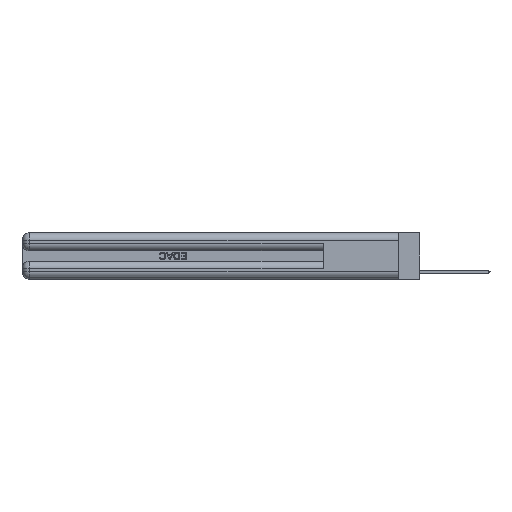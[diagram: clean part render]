
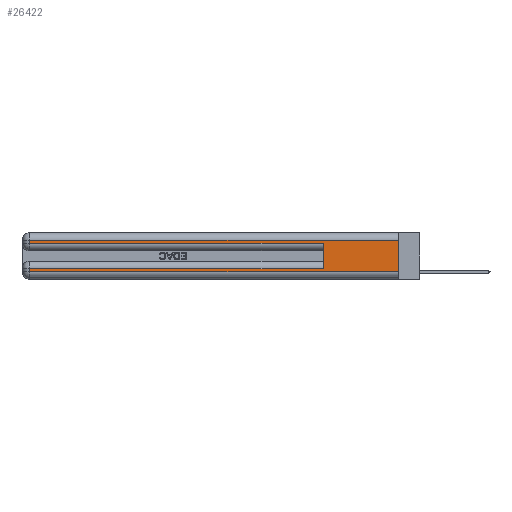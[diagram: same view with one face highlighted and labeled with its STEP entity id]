
A CAD part, left-side view. The second image highlights one B-rep face of the part: STEP entity #26422.
In plain terms, the highlighted planar face has unit normal (-1, 0, 0).
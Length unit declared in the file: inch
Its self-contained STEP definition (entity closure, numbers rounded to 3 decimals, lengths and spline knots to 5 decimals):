
#332 = ORIENTED_EDGE ( 'NONE', *, *, #34627, .T. ) ;
#1749 = CARTESIAN_POINT ( 'NONE',  ( 0., 2.94, 0.31 ) ) ;
#1881 = ORIENTED_EDGE ( 'NONE', *, *, #20156, .T. ) ;
#1884 = VERTEX_POINT ( 'NONE', #12785 ) ;
#2151 = ORIENTED_EDGE ( 'NONE', *, *, #9709, .T. ) ;
#2262 = CARTESIAN_POINT ( 'NONE',  ( 0., 2.94, 0.37 ) ) ;
#3121 = LINE ( 'NONE', #33482, #12870 ) ;
#4342 = VECTOR ( 'NONE', #13943, 39.37008 ) ;
#4448 = DIRECTION ( 'NONE',  ( 0., 0., -1. ) ) ;
#4853 = DIRECTION ( 'NONE',  ( 0., -1., 0. ) ) ;
#5162 = ORIENTED_EDGE ( 'NONE', *, *, #14232, .F. ) ;
#5972 = VERTEX_POINT ( 'NONE', #6393 ) ;
#6241 = VERTEX_POINT ( 'NONE', #8522 ) ;
#6393 = CARTESIAN_POINT ( 'NONE',  ( 0., 0.6, 0.085 ) ) ;
#7024 = VERTEX_POINT ( 'NONE', #1749 ) ;
#7501 = LINE ( 'NONE', #24125, #8134 ) ;
#7768 = CARTESIAN_POINT ( 'NONE',  ( 0., 0., 0.31 ) ) ;
#7909 = EDGE_LOOP ( 'NONE', ( #17252, #32436, #8553, #2151, #5162, #1881, #332, #27523 ) ) ;
#7910 = VECTOR ( 'NONE', #22847, 39.37008 ) ;
#8134 = VECTOR ( 'NONE', #8219, 39.37008 ) ;
#8219 = DIRECTION ( 'NONE',  ( 0., -1., 0. ) ) ;
#8522 = CARTESIAN_POINT ( 'NONE',  ( 0., 2.94, 0.285 ) ) ;
#8553 = ORIENTED_EDGE ( 'NONE', *, *, #19678, .T. ) ;
#9529 = CARTESIAN_POINT ( 'NONE',  ( 0., 0., 0.37 ) ) ;
#9709 = EDGE_CURVE ( 'NONE', #6241, #11532, #16618, .T. ) ;
#10298 = DIRECTION ( 'NONE',  ( 0., 1., 0. ) ) ;
#11532 = VERTEX_POINT ( 'NONE', #32826 ) ;
#12074 = FACE_OUTER_BOUND ( 'NONE', #7909, .T. ) ;
#12177 = LINE ( 'NONE', #31848, #17243 ) ;
#12514 = LINE ( 'NONE', #18135, #7910 ) ;
#12785 = CARTESIAN_POINT ( 'NONE',  ( 0., 0., 0.06 ) ) ;
#12870 = VECTOR ( 'NONE', #19405, 39.37008 ) ;
#13943 = DIRECTION ( 'NONE',  ( 0., 1., 0. ) ) ;
#14232 = EDGE_CURVE ( 'NONE', #5972, #11532, #3121, .T. ) ;
#14872 = VERTEX_POINT ( 'NONE', #17557 ) ;
#15787 = DIRECTION ( 'NONE',  ( 0., 0., -1. ) ) ;
#16210 = LINE ( 'NONE', #2262, #18440 ) ;
#16618 = LINE ( 'NONE', #32509, #30631 ) ;
#16631 = VERTEX_POINT ( 'NONE', #17161 ) ;
#17161 = CARTESIAN_POINT ( 'NONE',  ( 0., 2.94, 0.085 ) ) ;
#17243 = VECTOR ( 'NONE', #15787, 39.37008 ) ;
#17252 = ORIENTED_EDGE ( 'NONE', *, *, #24748, .F. ) ;
#17557 = CARTESIAN_POINT ( 'NONE',  ( 0., 2.94, 0.06 ) ) ;
#17682 = PLANE ( 'NONE',  #24805 ) ;
#18135 = CARTESIAN_POINT ( 'NONE',  ( 0., 2.94, 0.37 ) ) ;
#18204 = VERTEX_POINT ( 'NONE', #33874 ) ;
#18440 = VECTOR ( 'NONE', #21803, 39.37008 ) ;
#19405 = DIRECTION ( 'NONE',  ( 0., 0., 1. ) ) ;
#19549 = CARTESIAN_POINT ( 'NONE',  ( 0., 0., 0.085 ) ) ;
#19678 = EDGE_CURVE ( 'NONE', #7024, #6241, #16210, .T. ) ;
#20156 = EDGE_CURVE ( 'NONE', #5972, #16631, #33439, .T. ) ;
#21803 = DIRECTION ( 'NONE',  ( 0., 0., -1. ) ) ;
#22847 = DIRECTION ( 'NONE',  ( 0., 0., -1. ) ) ;
#23104 = DIRECTION ( 'NONE',  ( 1., 0., 0. ) ) ;
#24125 = CARTESIAN_POINT ( 'NONE',  ( 0., 0., 0.06 ) ) ;
#24748 = EDGE_CURVE ( 'NONE', #18204, #1884, #12177, .T. ) ;
#24805 = AXIS2_PLACEMENT_3D ( 'NONE', #9529, #23104, #4448 ) ;
#26422 = ADVANCED_FACE ( 'NONE', ( #12074 ), #17682, .F. ) ;
#27523 = ORIENTED_EDGE ( 'NONE', *, *, #28096, .T. ) ;
#28096 = EDGE_CURVE ( 'NONE', #14872, #1884, #7501, .T. ) ;
#29637 = LINE ( 'NONE', #7768, #31010 ) ;
#30631 = VECTOR ( 'NONE', #4853, 39.37008 ) ;
#31010 = VECTOR ( 'NONE', #10298, 39.37008 ) ;
#31848 = CARTESIAN_POINT ( 'NONE',  ( 0., 0., 0.37 ) ) ;
#32436 = ORIENTED_EDGE ( 'NONE', *, *, #35143, .T. ) ;
#32509 = CARTESIAN_POINT ( 'NONE',  ( 0., 0., 0.285 ) ) ;
#32826 = CARTESIAN_POINT ( 'NONE',  ( 0., 0.6, 0.285 ) ) ;
#33439 = LINE ( 'NONE', #19549, #4342 ) ;
#33482 = CARTESIAN_POINT ( 'NONE',  ( 0., 0.6, 0.145 ) ) ;
#33874 = CARTESIAN_POINT ( 'NONE',  ( 0., 0., 0.31 ) ) ;
#34627 = EDGE_CURVE ( 'NONE', #16631, #14872, #12514, .T. ) ;
#35143 = EDGE_CURVE ( 'NONE', #18204, #7024, #29637, .T. ) ;
